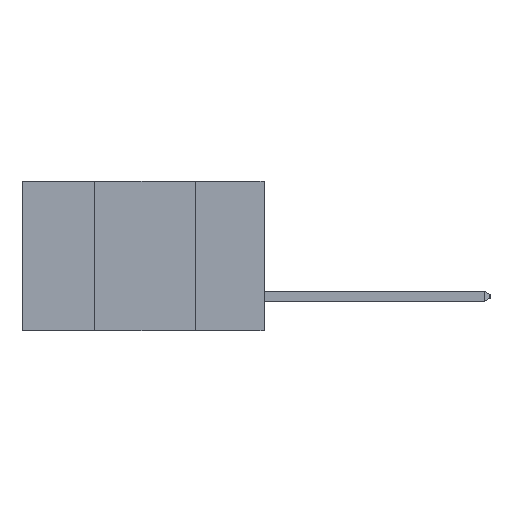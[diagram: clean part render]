
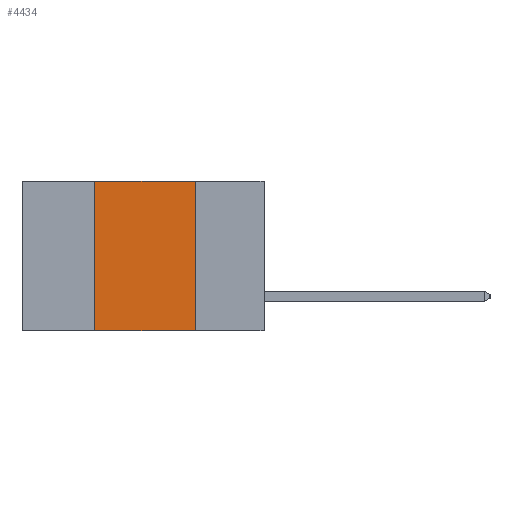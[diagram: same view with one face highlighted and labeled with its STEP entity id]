
A CAD part, left-side view. The second image highlights one B-rep face of the part: STEP entity #4434.
In plain terms, the highlighted planar face has unit normal (-1, 0, 0).
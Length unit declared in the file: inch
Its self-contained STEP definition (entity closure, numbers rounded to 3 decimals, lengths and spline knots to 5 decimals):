
#43 = VECTOR ( 'NONE', #8251, 39.37008 ) ;
#97 = CARTESIAN_POINT ( 'NONE',  ( 0., 0.42, 0. ) ) ;
#146 = ORIENTED_EDGE ( 'NONE', *, *, #919, .F. ) ;
#199 = LINE ( 'NONE', #4571, #7531 ) ;
#919 = EDGE_CURVE ( 'NONE', #1711, #9523, #8296, .T. ) ;
#1377 = DIRECTION ( 'NONE',  ( 0., 0., 1. ) ) ;
#1496 = DIRECTION ( 'NONE',  ( 0., -1., 0. ) ) ;
#1512 = CARTESIAN_POINT ( 'NONE',  ( 0., 0.6, -0.37 ) ) ;
#1711 = VERTEX_POINT ( 'NONE', #4747 ) ;
#2347 = EDGE_CURVE ( 'NONE', #9398, #11768, #10100, .T. ) ;
#2599 = EDGE_CURVE ( 'NONE', #9523, #9398, #199, .T. ) ;
#2854 = LINE ( 'NONE', #1512, #7494 ) ;
#3376 = VECTOR ( 'NONE', #1377, 39.37008 ) ;
#3674 = ORIENTED_EDGE ( 'NONE', *, *, #6530, .T. ) ;
#3955 = CARTESIAN_POINT ( 'NONE',  ( 0., 0.17, -0.37 ) ) ;
#4434 = ADVANCED_FACE ( 'NONE', ( #9065 ), #11047, .F. ) ;
#4571 = CARTESIAN_POINT ( 'NONE',  ( 0., 0.6, 0. ) ) ;
#4686 = DIRECTION ( 'NONE',  ( 0., -1., 0. ) ) ;
#4747 = CARTESIAN_POINT ( 'NONE',  ( 0., 0.42, -0.37 ) ) ;
#4986 = ORIENTED_EDGE ( 'NONE', *, *, #2599, .F. ) ;
#5553 = EDGE_LOOP ( 'NONE', ( #10942, #4986, #146, #3674 ) ) ;
#6427 = CARTESIAN_POINT ( 'NONE',  ( 0., 0.42, -0.37 ) ) ;
#6530 = EDGE_CURVE ( 'NONE', #1711, #11768, #2854, .T. ) ;
#7494 = VECTOR ( 'NONE', #1496, 39.37008 ) ;
#7531 = VECTOR ( 'NONE', #4686, 39.37008 ) ;
#8224 = AXIS2_PLACEMENT_3D ( 'NONE', #10085, #11298, #11285 ) ;
#8251 = DIRECTION ( 'NONE',  ( 0., 0., -1. ) ) ;
#8296 = LINE ( 'NONE', #6427, #3376 ) ;
#8776 = CARTESIAN_POINT ( 'NONE',  ( 0., 0.17, -0.37 ) ) ;
#9065 = FACE_OUTER_BOUND ( 'NONE', #5553, .T. ) ;
#9398 = VERTEX_POINT ( 'NONE', #10283 ) ;
#9523 = VERTEX_POINT ( 'NONE', #97 ) ;
#10085 = CARTESIAN_POINT ( 'NONE',  ( 0., 0.6, 0. ) ) ;
#10100 = LINE ( 'NONE', #3955, #43 ) ;
#10283 = CARTESIAN_POINT ( 'NONE',  ( 0., 0.17, 0. ) ) ;
#10942 = ORIENTED_EDGE ( 'NONE', *, *, #2347, .F. ) ;
#11047 = PLANE ( 'NONE',  #8224 ) ;
#11285 = DIRECTION ( 'NONE',  ( 0., 0., -1. ) ) ;
#11298 = DIRECTION ( 'NONE',  ( 1., 0., 0. ) ) ;
#11768 = VERTEX_POINT ( 'NONE', #8776 ) ;
